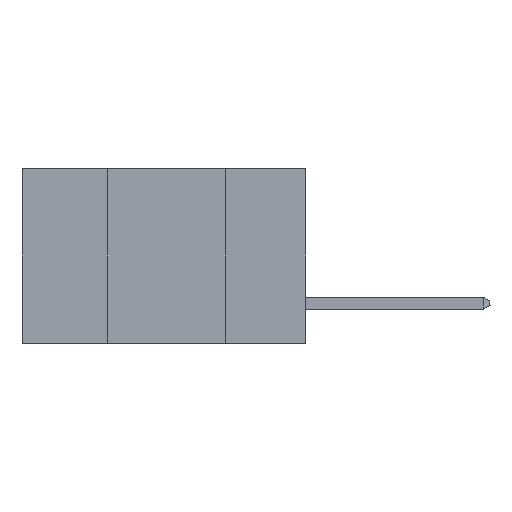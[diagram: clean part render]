
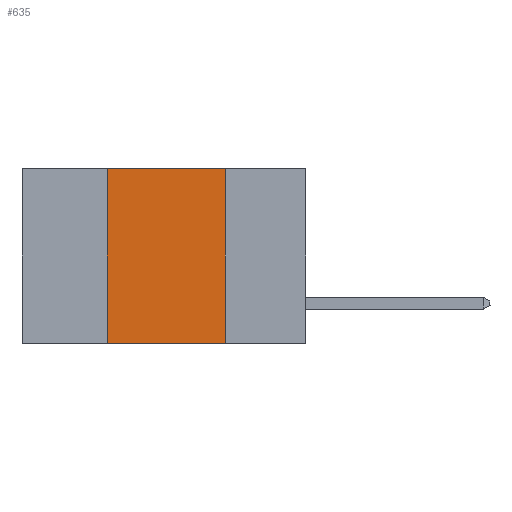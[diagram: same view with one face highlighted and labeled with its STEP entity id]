
A CAD part, left-side view. The second image highlights one B-rep face of the part: STEP entity #635.
In plain terms, the highlighted planar face has unit normal (-1, 0, 0).
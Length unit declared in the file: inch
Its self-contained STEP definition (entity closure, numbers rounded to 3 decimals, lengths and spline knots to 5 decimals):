
#355 = VERTEX_POINT ( 'NONE', #15324 ) ;
#635 = ADVANCED_FACE ( 'NONE', ( #3751 ), #20027, .F. ) ;
#981 = LINE ( 'NONE', #10387, #18892 ) ;
#1047 = ORIENTED_EDGE ( 'NONE', *, *, #28435, .F. ) ;
#2598 = DIRECTION ( 'NONE',  ( 0., 0., -1. ) ) ;
#3346 = DIRECTION ( 'NONE',  ( 0., 0., 1. ) ) ;
#3751 = FACE_OUTER_BOUND ( 'NONE', #27135, .T. ) ;
#4191 = DIRECTION ( 'NONE',  ( 0., -1., 0. ) ) ;
#4505 = AXIS2_PLACEMENT_3D ( 'NONE', #27802, #22793, #26276 ) ;
#7185 = CARTESIAN_POINT ( 'NONE',  ( 0., 0.6, -0.37 ) ) ;
#7454 = VERTEX_POINT ( 'NONE', #25463 ) ;
#8093 = LINE ( 'NONE', #15917, #19846 ) ;
#9066 = VECTOR ( 'NONE', #2598, 39.37008 ) ;
#9556 = CARTESIAN_POINT ( 'NONE',  ( 0., 0.17, 0. ) ) ;
#9667 = LINE ( 'NONE', #7185, #15203 ) ;
#10387 = CARTESIAN_POINT ( 'NONE',  ( 0., 0.42, 0. ) ) ;
#11257 = CARTESIAN_POINT ( 'NONE',  ( 0., 0.17, 0. ) ) ;
#15203 = VECTOR ( 'NONE', #25878, 39.37008 ) ;
#15324 = CARTESIAN_POINT ( 'NONE',  ( 0., 0.42, -0.37 ) ) ;
#15364 = LINE ( 'NONE', #9556, #9066 ) ;
#15917 = CARTESIAN_POINT ( 'NONE',  ( 0., 0.6, 0. ) ) ;
#18892 = VECTOR ( 'NONE', #3346, 39.37008 ) ;
#19570 = EDGE_CURVE ( 'NONE', #23922, #29250, #15364, .T. ) ;
#19846 = VECTOR ( 'NONE', #4191, 39.37008 ) ;
#20027 = PLANE ( 'NONE',  #4505 ) ;
#21092 = ORIENTED_EDGE ( 'NONE', *, *, #21111, .F. ) ;
#21111 = EDGE_CURVE ( 'NONE', #355, #7454, #981, .T. ) ;
#21915 = ORIENTED_EDGE ( 'NONE', *, *, #19570, .F. ) ;
#22793 = DIRECTION ( 'NONE',  ( 1., 0., 0. ) ) ;
#23922 = VERTEX_POINT ( 'NONE', #11257 ) ;
#25463 = CARTESIAN_POINT ( 'NONE',  ( 0., 0.42, 0. ) ) ;
#25878 = DIRECTION ( 'NONE',  ( 0., -1., 0. ) ) ;
#25965 = CARTESIAN_POINT ( 'NONE',  ( 0., 0.17, -0.37 ) ) ;
#26276 = DIRECTION ( 'NONE',  ( 0., 0., -1. ) ) ;
#27135 = EDGE_LOOP ( 'NONE', ( #21915, #1047, #21092, #27625 ) ) ;
#27300 = EDGE_CURVE ( 'NONE', #355, #29250, #9667, .T. ) ;
#27625 = ORIENTED_EDGE ( 'NONE', *, *, #27300, .T. ) ;
#27802 = CARTESIAN_POINT ( 'NONE',  ( 0., 0.6, 0. ) ) ;
#28435 = EDGE_CURVE ( 'NONE', #7454, #23922, #8093, .T. ) ;
#29250 = VERTEX_POINT ( 'NONE', #25965 ) ;
